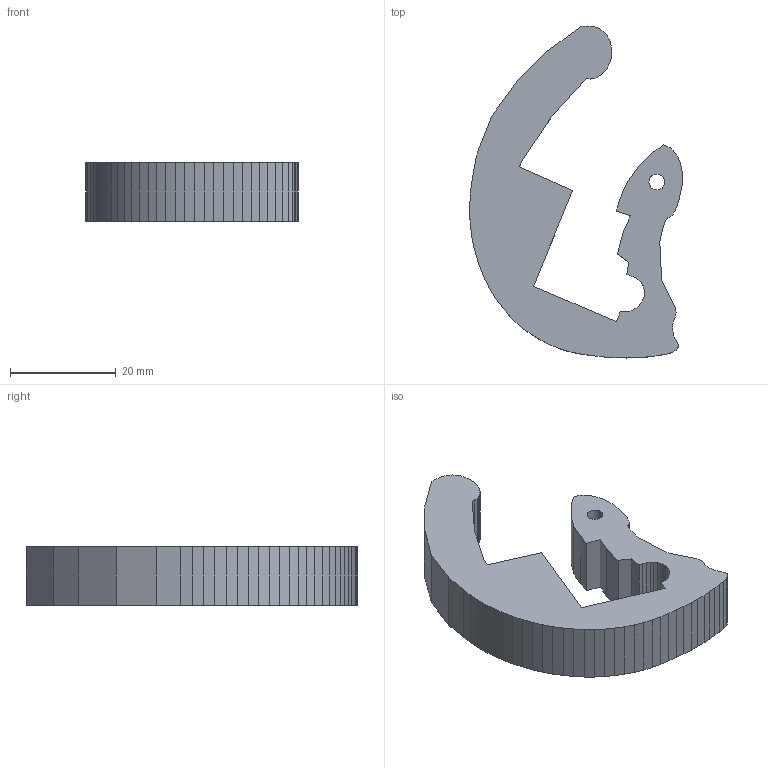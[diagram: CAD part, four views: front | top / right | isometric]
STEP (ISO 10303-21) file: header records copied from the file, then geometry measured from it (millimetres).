
FILE_DESCRIPTION((''),'2;1');
FILE_NAME('trigger.stp','2013-08-15T20:15:26',('mrfr'),(''),'Autodesk Inventor 2013','Autodesk Inventor 2013','');
FILE_SCHEMA(('AUTOMOTIVE_DESIGN { 1 0 10303 214 1 1 1 1 }'));
Length unit declared in the file: millimetre
Products named in the file (1): trigger
Bounding box: 40.26 x 62.82 x 11 mm (x, y, z)
Volume: 12423.1 mm3; surface area: 5349.4 mm2
Topology: 1 solids, 1 shells, 133 faces, 393 edges, 262 vertices
Faces by surface type: plane 129, cylinder 4
Full cylindrical faces by diameter (mm): 3 x1
Entity records: 4380 total; most frequent: CARTESIAN_POINT 788, ORIENTED_EDGE 784, DIRECTION 668, EDGE_CURVE 392, VECTOR 384, LINE 384, VERTEX_POINT 262, AXIS2_PLACEMENT_3D 142
